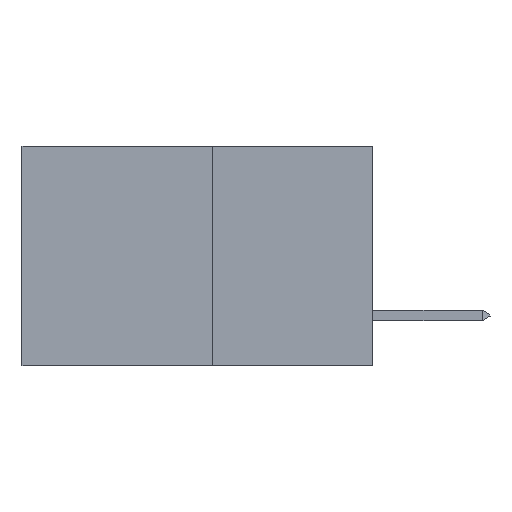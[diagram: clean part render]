
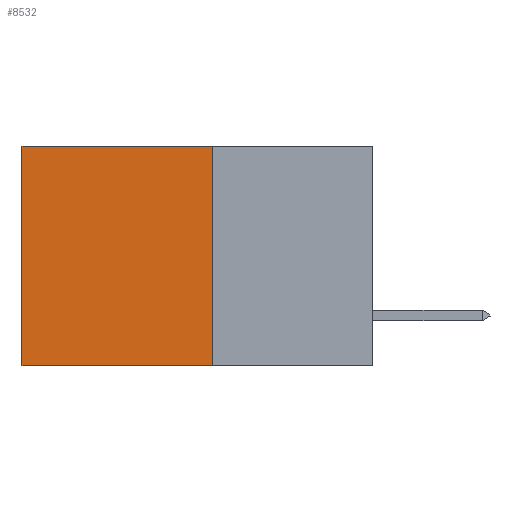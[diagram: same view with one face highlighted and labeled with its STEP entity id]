
A CAD part, left-side view. The second image highlights one B-rep face of the part: STEP entity #8532.
In plain terms, the highlighted planar face has unit normal (-1, 0, 0).
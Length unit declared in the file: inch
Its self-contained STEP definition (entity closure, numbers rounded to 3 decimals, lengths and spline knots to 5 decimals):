
#392 = VERTEX_POINT ( 'NONE', #2962 ) ;
#680 = ORIENTED_EDGE ( 'NONE', *, *, #18404, .T. ) ;
#1339 = VECTOR ( 'NONE', #12243, 39.37008 ) ;
#2181 = FACE_OUTER_BOUND ( 'NONE', #10427, .T. ) ;
#2374 = LINE ( 'NONE', #16404, #14901 ) ;
#2423 = CARTESIAN_POINT ( 'NONE',  ( 0.277, 0.27, -0.37 ) ) ;
#2835 = CARTESIAN_POINT ( 'NONE',  ( 0.277, 0.59, -0.37 ) ) ;
#2962 = CARTESIAN_POINT ( 'NONE',  ( 0.277, 0.59, 0. ) ) ;
#3387 = ORIENTED_EDGE ( 'NONE', *, *, #9584, .F. ) ;
#3773 = CARTESIAN_POINT ( 'NONE',  ( 0.277, 0.27, -0.37 ) ) ;
#4132 = LINE ( 'NONE', #8043, #20783 ) ;
#5119 = DIRECTION ( 'NONE',  ( 0., 1., 0. ) ) ;
#6149 = CARTESIAN_POINT ( 'NONE',  ( 0.277, 0.59, -0.37 ) ) ;
#6850 = EDGE_CURVE ( 'NONE', #392, #18125, #13869, .T. ) ;
#6919 = EDGE_CURVE ( 'NONE', #19272, #18125, #4132, .T. ) ;
#7451 = AXIS2_PLACEMENT_3D ( 'NONE', #15642, #20440, #10922 ) ;
#8043 = CARTESIAN_POINT ( 'NONE',  ( 0.277, 0.27, -0.37 ) ) ;
#8532 = ADVANCED_FACE ( 'NONE', ( #2181 ), #18862, .F. ) ;
#9542 = VECTOR ( 'NONE', #11173, 39.37008 ) ;
#9584 = EDGE_CURVE ( 'NONE', #13393, #19272, #13442, .T. ) ;
#9696 = DIRECTION ( 'NONE',  ( 0., 1., 0. ) ) ;
#10427 = EDGE_LOOP ( 'NONE', ( #10734, #16165, #3387, #680 ) ) ;
#10734 = ORIENTED_EDGE ( 'NONE', *, *, #6850, .T. ) ;
#10922 = DIRECTION ( 'NONE',  ( 0., 0., -1. ) ) ;
#11173 = DIRECTION ( 'NONE',  ( 0., 0., -1. ) ) ;
#12243 = DIRECTION ( 'NONE',  ( 0., 0., -1. ) ) ;
#13393 = VERTEX_POINT ( 'NONE', #21020 ) ;
#13442 = LINE ( 'NONE', #2423, #1339 ) ;
#13869 = LINE ( 'NONE', #6149, #9542 ) ;
#14901 = VECTOR ( 'NONE', #5119, 39.37008 ) ;
#15642 = CARTESIAN_POINT ( 'NONE',  ( 0.277, 0.27, -0.37 ) ) ;
#16165 = ORIENTED_EDGE ( 'NONE', *, *, #6919, .F. ) ;
#16404 = CARTESIAN_POINT ( 'NONE',  ( 0.277, 0.27, 0. ) ) ;
#18125 = VERTEX_POINT ( 'NONE', #2835 ) ;
#18404 = EDGE_CURVE ( 'NONE', #13393, #392, #2374, .T. ) ;
#18862 = PLANE ( 'NONE',  #7451 ) ;
#19272 = VERTEX_POINT ( 'NONE', #3773 ) ;
#20440 = DIRECTION ( 'NONE',  ( 1., 0., 0. ) ) ;
#20783 = VECTOR ( 'NONE', #9696, 39.37008 ) ;
#21020 = CARTESIAN_POINT ( 'NONE',  ( 0.277, 0.27, 0. ) ) ;
